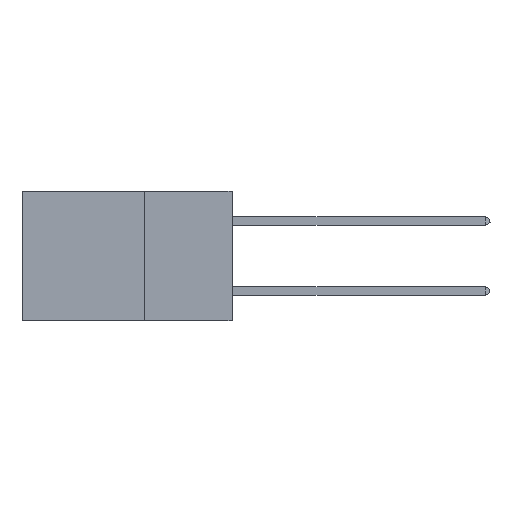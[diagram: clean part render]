
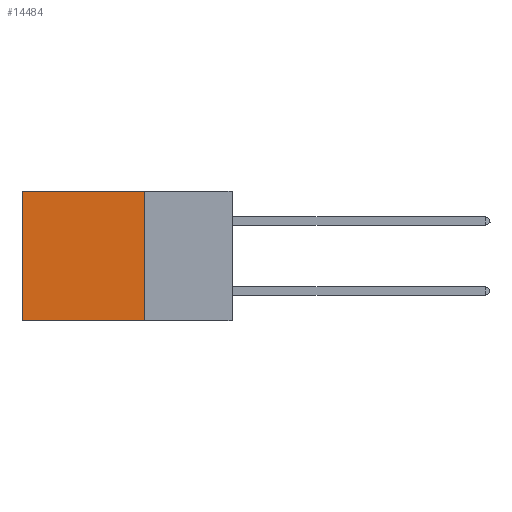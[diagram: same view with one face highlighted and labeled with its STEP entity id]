
A CAD part, left-side view. The second image highlights one B-rep face of the part: STEP entity #14484.
In plain terms, the highlighted planar face has unit normal (-1, 0, 0).
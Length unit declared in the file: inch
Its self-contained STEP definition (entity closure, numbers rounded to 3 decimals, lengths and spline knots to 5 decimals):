
#1301 = ORIENTED_EDGE ( 'NONE', *, *, #8814, .F. ) ;
#1405 = CARTESIAN_POINT ( 'NONE',  ( 0.2875, 0.25, 0. ) ) ;
#2470 = VECTOR ( 'NONE', #9410, 39.37008 ) ;
#2674 = CARTESIAN_POINT ( 'NONE',  ( 0.2875, 0.6, -0.37 ) ) ;
#3183 = DIRECTION ( 'NONE',  ( 0., 0., -1. ) ) ;
#3541 = LINE ( 'NONE', #9905, #15087 ) ;
#3647 = VERTEX_POINT ( 'NONE', #15992 ) ;
#3770 = CARTESIAN_POINT ( 'NONE',  ( 0.2875, 0.25, -0.37 ) ) ;
#4112 = LINE ( 'NONE', #1405, #2470 ) ;
#4225 = ORIENTED_EDGE ( 'NONE', *, *, #11957, .T. ) ;
#4633 = DIRECTION ( 'NONE',  ( 0., 0., -1. ) ) ;
#5807 = CARTESIAN_POINT ( 'NONE',  ( 0.2875, 0.25, 0. ) ) ;
#6230 = EDGE_LOOP ( 'NONE', ( #4225, #6499, #1301, #10752 ) ) ;
#6274 = FACE_OUTER_BOUND ( 'NONE', #6230, .T. ) ;
#6499 = ORIENTED_EDGE ( 'NONE', *, *, #12589, .F. ) ;
#6816 = DIRECTION ( 'NONE',  ( 0., 0., -1. ) ) ;
#6908 = LINE ( 'NONE', #9434, #13427 ) ;
#8814 = EDGE_CURVE ( 'NONE', #3647, #14004, #9893, .T. ) ;
#9410 = DIRECTION ( 'NONE',  ( 0., 1., 0. ) ) ;
#9434 = CARTESIAN_POINT ( 'NONE',  ( 0.2875, 0.6, 0. ) ) ;
#9893 = LINE ( 'NONE', #5807, #16442 ) ;
#9905 = CARTESIAN_POINT ( 'NONE',  ( 0.2875, 0.25, -0.37 ) ) ;
#10185 = PLANE ( 'NONE',  #11010 ) ;
#10752 = ORIENTED_EDGE ( 'NONE', *, *, #14650, .T. ) ;
#11010 = AXIS2_PLACEMENT_3D ( 'NONE', #11563, #15446, #4633 ) ;
#11563 = CARTESIAN_POINT ( 'NONE',  ( 0.2875, 0.25, 0. ) ) ;
#11957 = EDGE_CURVE ( 'NONE', #14285, #15158, #6908, .T. ) ;
#12184 = CARTESIAN_POINT ( 'NONE',  ( 0.2875, 0.6, 0. ) ) ;
#12589 = EDGE_CURVE ( 'NONE', #14004, #15158, #3541, .T. ) ;
#13427 = VECTOR ( 'NONE', #6816, 39.37008 ) ;
#13794 = DIRECTION ( 'NONE',  ( 0., 1., 0. ) ) ;
#14004 = VERTEX_POINT ( 'NONE', #3770 ) ;
#14285 = VERTEX_POINT ( 'NONE', #12184 ) ;
#14484 = ADVANCED_FACE ( 'NONE', ( #6274 ), #10185, .F. ) ;
#14650 = EDGE_CURVE ( 'NONE', #3647, #14285, #4112, .T. ) ;
#15087 = VECTOR ( 'NONE', #13794, 39.37008 ) ;
#15158 = VERTEX_POINT ( 'NONE', #2674 ) ;
#15446 = DIRECTION ( 'NONE',  ( 1., 0., 0. ) ) ;
#15992 = CARTESIAN_POINT ( 'NONE',  ( 0.2875, 0.25, 0. ) ) ;
#16442 = VECTOR ( 'NONE', #3183, 39.37008 ) ;
